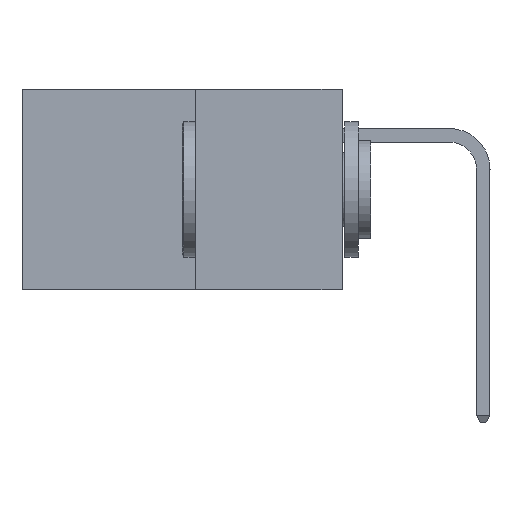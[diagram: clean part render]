
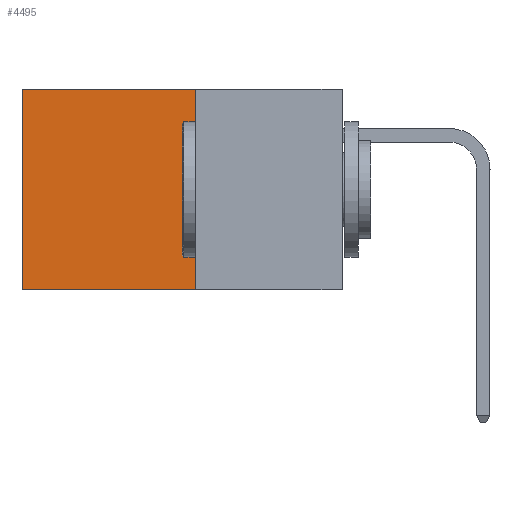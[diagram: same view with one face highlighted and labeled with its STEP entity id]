
A CAD part, left-side view. The second image highlights one B-rep face of the part: STEP entity #4495.
In plain terms, the highlighted planar face has unit normal (-1, 0, 0).
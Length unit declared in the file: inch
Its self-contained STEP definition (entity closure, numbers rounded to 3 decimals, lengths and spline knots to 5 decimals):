
#123 = CARTESIAN_POINT ( 'NONE',  ( 0.277, 0.59, -0.37 ) ) ;
#544 = VERTEX_POINT ( 'NONE', #8061 ) ;
#856 = DIRECTION ( 'NONE',  ( 0., 0., -1. ) ) ;
#1367 = EDGE_LOOP ( 'NONE', ( #2822, #7444, #9549, #3347 ) ) ;
#1479 = VERTEX_POINT ( 'NONE', #10040 ) ;
#1572 = CARTESIAN_POINT ( 'NONE',  ( 0.277, 0.27, -0.37 ) ) ;
#1939 = AXIS2_PLACEMENT_3D ( 'NONE', #1572, #2289, #856 ) ;
#2289 = DIRECTION ( 'NONE',  ( 1., 0., 0. ) ) ;
#2743 = PLANE ( 'NONE',  #1939 ) ;
#2758 = VECTOR ( 'NONE', #3759, 39.37008 ) ;
#2822 = ORIENTED_EDGE ( 'NONE', *, *, #3587, .T. ) ;
#2899 = EDGE_CURVE ( 'NONE', #1479, #544, #9734, .T. ) ;
#3154 = CARTESIAN_POINT ( 'NONE',  ( 0.277, 0.27, -0.37 ) ) ;
#3347 = ORIENTED_EDGE ( 'NONE', *, *, #2899, .T. ) ;
#3587 = EDGE_CURVE ( 'NONE', #544, #8214, #9129, .T. ) ;
#3759 = DIRECTION ( 'NONE',  ( 0., 1., 0. ) ) ;
#4495 = ADVANCED_FACE ( 'NONE', ( #10608 ), #2743, .F. ) ;
#5147 = DIRECTION ( 'NONE',  ( 0., 0., -1. ) ) ;
#7373 = LINE ( 'NONE', #10750, #9489 ) ;
#7444 = ORIENTED_EDGE ( 'NONE', *, *, #7473, .F. ) ;
#7473 = EDGE_CURVE ( 'NONE', #10720, #8214, #10443, .T. ) ;
#8061 = CARTESIAN_POINT ( 'NONE',  ( 0.277, 0.59, 0. ) ) ;
#8214 = VERTEX_POINT ( 'NONE', #9083 ) ;
#8238 = DIRECTION ( 'NONE',  ( 0., 0., -1. ) ) ;
#8346 = EDGE_CURVE ( 'NONE', #1479, #10720, #7373, .T. ) ;
#8385 = DIRECTION ( 'NONE',  ( 0., 1., 0. ) ) ;
#8477 = VECTOR ( 'NONE', #8385, 39.37008 ) ;
#9083 = CARTESIAN_POINT ( 'NONE',  ( 0.277, 0.59, -0.37 ) ) ;
#9129 = LINE ( 'NONE', #123, #10853 ) ;
#9306 = CARTESIAN_POINT ( 'NONE',  ( 0.277, 0.27, -0.37 ) ) ;
#9353 = CARTESIAN_POINT ( 'NONE',  ( 0.277, 0.27, 0. ) ) ;
#9489 = VECTOR ( 'NONE', #5147, 39.37008 ) ;
#9549 = ORIENTED_EDGE ( 'NONE', *, *, #8346, .F. ) ;
#9734 = LINE ( 'NONE', #9353, #2758 ) ;
#10040 = CARTESIAN_POINT ( 'NONE',  ( 0.277, 0.27, 0. ) ) ;
#10443 = LINE ( 'NONE', #3154, #8477 ) ;
#10608 = FACE_OUTER_BOUND ( 'NONE', #1367, .T. ) ;
#10720 = VERTEX_POINT ( 'NONE', #9306 ) ;
#10750 = CARTESIAN_POINT ( 'NONE',  ( 0.277, 0.27, -0.37 ) ) ;
#10853 = VECTOR ( 'NONE', #8238, 39.37008 ) ;
